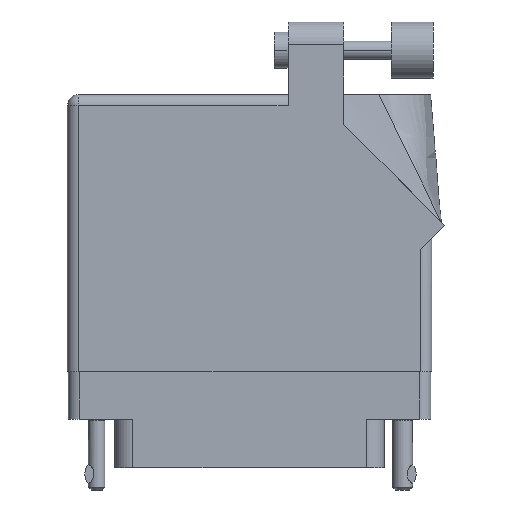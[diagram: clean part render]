
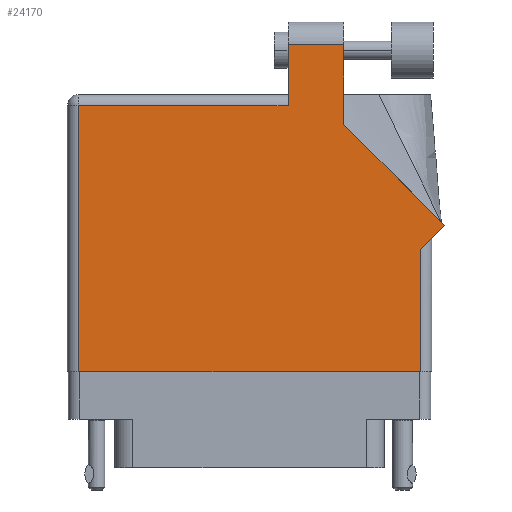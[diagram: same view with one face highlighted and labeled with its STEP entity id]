
A CAD part, front view. The second image highlights one B-rep face of the part: STEP entity #24170.
In plain terms, the highlighted face is planar.
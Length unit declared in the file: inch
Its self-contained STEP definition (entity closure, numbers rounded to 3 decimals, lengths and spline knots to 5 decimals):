
#1130 = VERTEX_POINT ( 'NONE', #43395 ) ;
#1660 = CARTESIAN_POINT ( 'NONE',  ( 1.524, 1.36442, 0. ) ) ;
#2427 = VECTOR ( 'NONE', #3593, 39.37008 ) ;
#2701 = EDGE_CURVE ( 'NONE', #12405, #22433, #29345, .T. ) ;
#2784 = DIRECTION ( 'NONE',  ( -1., 0., 0. ) ) ;
#3593 = DIRECTION ( 'NONE',  ( 0., -1., 0. ) ) ;
#3916 = VERTEX_POINT ( 'NONE', #47723 ) ;
#4468 = DIRECTION ( 'NONE',  ( -0.707, 0.707, 0. ) ) ;
#4645 = CARTESIAN_POINT ( 'NONE',  ( 2.01, 0.737, 0. ) ) ;
#6739 = VECTOR ( 'NONE', #24607, 39.37008 ) ;
#6912 = CARTESIAN_POINT ( 'NONE',  ( 1.217, 1.468, 0. ) ) ;
#7172 = ORIENTED_EDGE ( 'NONE', *, *, #24089, .T. ) ;
#8648 = CARTESIAN_POINT ( 'NONE',  ( 1.217, 1.53, 0. ) ) ;
#9344 = EDGE_LOOP ( 'NONE', ( #21387, #24197, #30417, #29189, #7172, #39631, #47560, #12448, #24935 ) ) ;
#10808 = CARTESIAN_POINT ( 'NONE',  ( 0., 1.468, 0. ) ) ;
#12405 = VERTEX_POINT ( 'NONE', #1660 ) ;
#12448 = ORIENTED_EDGE ( 'NONE', *, *, #26743, .T. ) ;
#14119 = LINE ( 'NONE', #8648, #2427 ) ;
#15700 = DIRECTION ( 'NONE',  ( -1., 0., 0. ) ) ;
#16200 = VERTEX_POINT ( 'NONE', #23878 ) ;
#17113 = EDGE_CURVE ( 'NONE', #39938, #1130, #36299, .T. ) ;
#17384 = LINE ( 'NONE', #45294, #26119 ) ;
#17809 = VECTOR ( 'NONE', #15700, 39.37008 ) ;
#18201 = VECTOR ( 'NONE', #36881, 39.37008 ) ;
#18829 = DIRECTION ( 'NONE',  ( 1., 0., 0. ) ) ;
#19270 = DIRECTION ( 'NONE',  ( 0.707, 0.707, 0. ) ) ;
#19743 = EDGE_CURVE ( 'NONE', #22433, #16200, #42815, .T. ) ;
#20026 = CARTESIAN_POINT ( 'NONE',  ( 0.062, 0., 0. ) ) ;
#20897 = LINE ( 'NONE', #41084, #29095 ) ;
#21162 = PLANE ( 'NONE',  #27501 ) ;
#21387 = ORIENTED_EDGE ( 'NONE', *, *, #2701, .T. ) ;
#22433 = VERTEX_POINT ( 'NONE', #32457 ) ;
#23323 = VERTEX_POINT ( 'NONE', #42695 ) ;
#23760 = DIRECTION ( 'NONE',  ( 0., -1., 0. ) ) ;
#23878 = CARTESIAN_POINT ( 'NONE',  ( 1.217, 1.805, 0. ) ) ;
#24089 = EDGE_CURVE ( 'NONE', #1130, #44181, #32083, .T. ) ;
#24170 = ADVANCED_FACE ( 'NONE', ( #43718 ), #21162, .F. ) ;
#24197 = ORIENTED_EDGE ( 'NONE', *, *, #19743, .T. ) ;
#24595 = VERTEX_POINT ( 'NONE', #38689 ) ;
#24607 = DIRECTION ( 'NONE',  ( 0., 1., 0. ) ) ;
#24935 = ORIENTED_EDGE ( 'NONE', *, *, #25144, .T. ) ;
#25144 = EDGE_CURVE ( 'NONE', #23323, #12405, #20897, .T. ) ;
#26119 = VECTOR ( 'NONE', #18829, 39.37008 ) ;
#26743 = EDGE_CURVE ( 'NONE', #3916, #23323, #45731, .T. ) ;
#27501 = AXIS2_PLACEMENT_3D ( 'NONE', #36325, #47125, #2784 ) ;
#28029 = VECTOR ( 'NONE', #23760, 39.37008 ) ;
#28847 = CARTESIAN_POINT ( 'NONE',  ( 1.948, 0.737, 0. ) ) ;
#29095 = VECTOR ( 'NONE', #4468, 39.37008 ) ;
#29189 = ORIENTED_EDGE ( 'NONE', *, *, #17113, .T. ) ;
#29305 = VECTOR ( 'NONE', #46927, 39.37008 ) ;
#29345 = LINE ( 'NONE', #39498, #29305 ) ;
#30417 = ORIENTED_EDGE ( 'NONE', *, *, #34165, .T. ) ;
#32083 = LINE ( 'NONE', #20026, #28029 ) ;
#32457 = CARTESIAN_POINT ( 'NONE',  ( 1.524, 1.805, 0. ) ) ;
#32743 = EDGE_CURVE ( 'NONE', #44181, #24595, #17384, .T. ) ;
#33466 = CARTESIAN_POINT ( 'NONE',  ( 1.217, 1.805, 0. ) ) ;
#34165 = EDGE_CURVE ( 'NONE', #16200, #39938, #14119, .T. ) ;
#36299 = LINE ( 'NONE', #10808, #18201 ) ;
#36325 = CARTESIAN_POINT ( 'NONE',  ( 0., 1.53, 0. ) ) ;
#36435 = LINE ( 'NONE', #28847, #6739 ) ;
#36881 = DIRECTION ( 'NONE',  ( -1., 0., 0. ) ) ;
#37148 = CARTESIAN_POINT ( 'NONE',  ( 0.062, 0., 0. ) ) ;
#38188 = VECTOR ( 'NONE', #19270, 39.37008 ) ;
#38689 = CARTESIAN_POINT ( 'NONE',  ( 1.948, 0., 0. ) ) ;
#39498 = CARTESIAN_POINT ( 'NONE',  ( 1.524, 1.36442, 0. ) ) ;
#39631 = ORIENTED_EDGE ( 'NONE', *, *, #32743, .T. ) ;
#39938 = VERTEX_POINT ( 'NONE', #6912 ) ;
#41084 = CARTESIAN_POINT ( 'NONE',  ( 2.08071, 0.80771, 0. ) ) ;
#42695 = CARTESIAN_POINT ( 'NONE',  ( 2.08071, 0.80771, 0. ) ) ;
#42815 = LINE ( 'NONE', #33466, #17809 ) ;
#43395 = CARTESIAN_POINT ( 'NONE',  ( 0.062, 1.468, 0. ) ) ;
#43718 = FACE_OUTER_BOUND ( 'NONE', #9344, .T. ) ;
#44181 = VERTEX_POINT ( 'NONE', #37148 ) ;
#45294 = CARTESIAN_POINT ( 'NONE',  ( 0., 0., 0. ) ) ;
#45731 = LINE ( 'NONE', #4645, #38188 ) ;
#46927 = DIRECTION ( 'NONE',  ( 0., 1., 0. ) ) ;
#46972 = EDGE_CURVE ( 'NONE', #24595, #3916, #36435, .T. ) ;
#47125 = DIRECTION ( 'NONE',  ( 0., 0., -1. ) ) ;
#47560 = ORIENTED_EDGE ( 'NONE', *, *, #46972, .T. ) ;
#47723 = CARTESIAN_POINT ( 'NONE',  ( 1.948, 0.675, 0. ) ) ;
